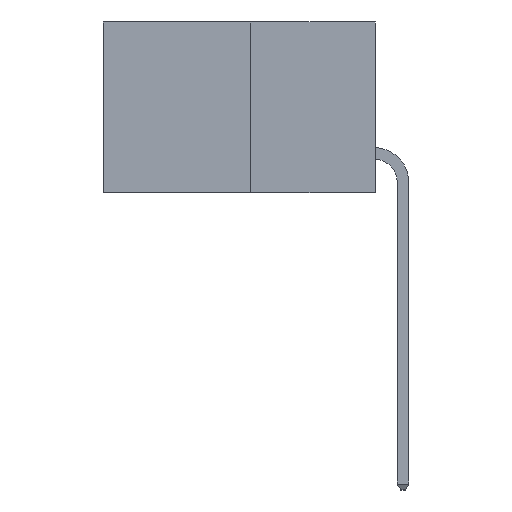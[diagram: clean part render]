
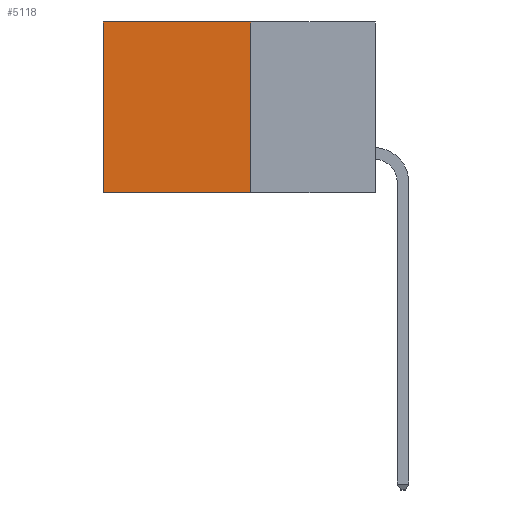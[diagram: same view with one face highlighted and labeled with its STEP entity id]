
A CAD part, left-side view. The second image highlights one B-rep face of the part: STEP entity #5118.
In plain terms, the highlighted planar face has unit normal (-1, 0, 0).
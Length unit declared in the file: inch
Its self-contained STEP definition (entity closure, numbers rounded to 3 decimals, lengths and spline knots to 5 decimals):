
#307 = VECTOR ( 'NONE', #7760, 39.37008 ) ;
#389 = AXIS2_PLACEMENT_3D ( 'NONE', #2684, #2675, #2654 ) ;
#556 = DIRECTION ( 'NONE',  ( 0., 1., 0. ) ) ;
#623 = CARTESIAN_POINT ( 'NONE',  ( 0.277, 0.27, -0.37 ) ) ;
#733 = CARTESIAN_POINT ( 'NONE',  ( 0.277, 0.59, -0.37 ) ) ;
#877 = EDGE_CURVE ( 'NONE', #5967, #5243, #2336, .T. ) ;
#939 = LINE ( 'NONE', #623, #6263 ) ;
#1045 = CARTESIAN_POINT ( 'NONE',  ( 0.277, 0.59, -0.37 ) ) ;
#1069 = VECTOR ( 'NONE', #7503, 39.37008 ) ;
#1720 = CARTESIAN_POINT ( 'NONE',  ( 0.277, 0.27, -0.37 ) ) ;
#2112 = CARTESIAN_POINT ( 'NONE',  ( 0.277, 0.27, 0. ) ) ;
#2320 = VERTEX_POINT ( 'NONE', #2112 ) ;
#2336 = LINE ( 'NONE', #733, #307 ) ;
#2453 = EDGE_LOOP ( 'NONE', ( #7922, #6188, #6777, #7983 ) ) ;
#2654 = DIRECTION ( 'NONE',  ( 0., 0., -1. ) ) ;
#2675 = DIRECTION ( 'NONE',  ( 1., 0., 0. ) ) ;
#2684 = CARTESIAN_POINT ( 'NONE',  ( 0.277, 0.27, -0.37 ) ) ;
#2829 = PLANE ( 'NONE',  #389 ) ;
#2969 = LINE ( 'NONE', #5530, #7982 ) ;
#3425 = EDGE_CURVE ( 'NONE', #2320, #5967, #2969, .T. ) ;
#4255 = CARTESIAN_POINT ( 'NONE',  ( 0.277, 0.59, 0. ) ) ;
#4853 = LINE ( 'NONE', #5754, #1069 ) ;
#5118 = ADVANCED_FACE ( 'NONE', ( #8350 ), #2829, .F. ) ;
#5243 = VERTEX_POINT ( 'NONE', #1045 ) ;
#5357 = DIRECTION ( 'NONE',  ( 0., 1., 0. ) ) ;
#5530 = CARTESIAN_POINT ( 'NONE',  ( 0.277, 0.27, 0. ) ) ;
#5754 = CARTESIAN_POINT ( 'NONE',  ( 0.277, 0.27, -0.37 ) ) ;
#5967 = VERTEX_POINT ( 'NONE', #4255 ) ;
#6188 = ORIENTED_EDGE ( 'NONE', *, *, #7436, .F. ) ;
#6263 = VECTOR ( 'NONE', #556, 39.37008 ) ;
#6777 = ORIENTED_EDGE ( 'NONE', *, *, #7649, .F. ) ;
#7436 = EDGE_CURVE ( 'NONE', #8014, #5243, #939, .T. ) ;
#7503 = DIRECTION ( 'NONE',  ( 0., 0., -1. ) ) ;
#7649 = EDGE_CURVE ( 'NONE', #2320, #8014, #4853, .T. ) ;
#7760 = DIRECTION ( 'NONE',  ( 0., 0., -1. ) ) ;
#7922 = ORIENTED_EDGE ( 'NONE', *, *, #877, .T. ) ;
#7982 = VECTOR ( 'NONE', #5357, 39.37008 ) ;
#7983 = ORIENTED_EDGE ( 'NONE', *, *, #3425, .T. ) ;
#8014 = VERTEX_POINT ( 'NONE', #1720 ) ;
#8350 = FACE_OUTER_BOUND ( 'NONE', #2453, .T. ) ;
